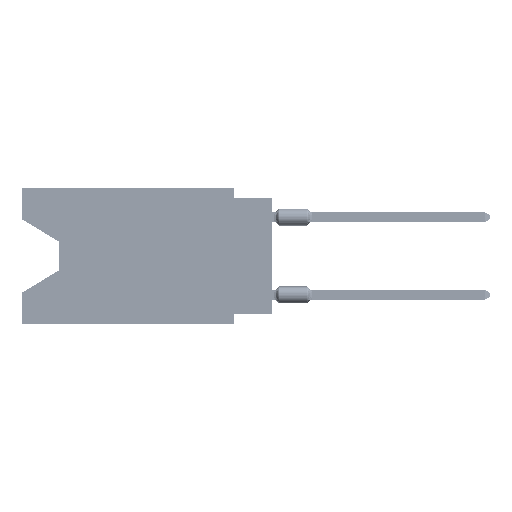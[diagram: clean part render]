
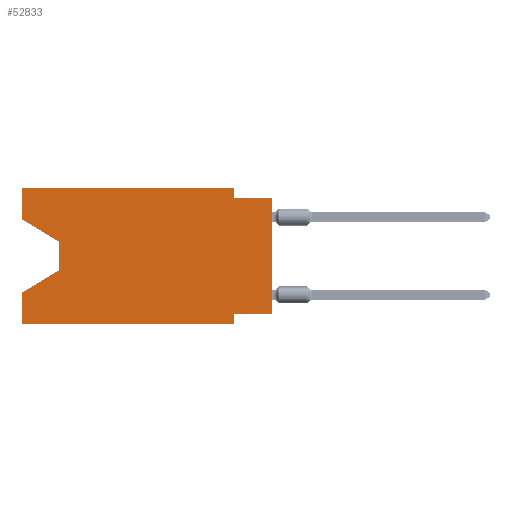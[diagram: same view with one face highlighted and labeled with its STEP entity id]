
A CAD part, left-side view. The second image highlights one B-rep face of the part: STEP entity #52833.
In plain terms, the highlighted planar face has unit normal (-1, 0, 0).
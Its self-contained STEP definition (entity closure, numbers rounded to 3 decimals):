
#71 = CARTESIAN_POINT ( 'NONE',  ( 0., 2.54, 0. ) ) ;
#236 = ORIENTED_EDGE ( 'NONE', *, *, #47545, .F. ) ;
#617 = VERTEX_POINT ( 'NONE', #4711 ) ;
#1688 = VECTOR ( 'NONE', #77916, 1000. ) ;
#2017 = EDGE_CURVE ( 'NONE', #23931, #95659, #14668, .T. ) ;
#2189 = LINE ( 'NONE', #18278, #55509 ) ;
#2536 = EDGE_CURVE ( 'NONE', #5876, #23931, #67046, .T. ) ;
#2810 = VECTOR ( 'NONE', #63174, 1000. ) ;
#3222 = VECTOR ( 'NONE', #25770, 1000. ) ;
#4711 = CARTESIAN_POINT ( 'NONE',  ( 0., 13.97, -5.385 ) ) ;
#5492 = EDGE_LOOP ( 'NONE', ( #47874, #43625, #38110, #98018, #96078, #26086, #236, #100570, #89663, #18626, #103654, #66525 ) ) ;
#5876 = VERTEX_POINT ( 'NONE', #17635 ) ;
#9688 = CARTESIAN_POINT ( 'NONE',  ( 0., 2.54, -8.89 ) ) ;
#13386 = CARTESIAN_POINT ( 'NONE',  ( 0., 16.383, 0. ) ) ;
#14668 = LINE ( 'NONE', #91004, #31913 ) ;
#17483 = CARTESIAN_POINT ( 'NONE',  ( 0., 0., -8.255 ) ) ;
#17635 = CARTESIAN_POINT ( 'NONE',  ( 0., 2.54, 0. ) ) ;
#18177 = CARTESIAN_POINT ( 'NONE',  ( 0., 16.383, -8.89 ) ) ;
#18278 = CARTESIAN_POINT ( 'NONE',  ( 0., 13.97, -3.505 ) ) ;
#18626 = ORIENTED_EDGE ( 'NONE', *, *, #2536, .F. ) ;
#18951 = EDGE_CURVE ( 'NONE', #60144, #62199, #61837, .T. ) ;
#20106 = EDGE_CURVE ( 'NONE', #58597, #37844, #100655, .T. ) ;
#23905 = DIRECTION ( 'NONE',  ( 0., 0., -1. ) ) ;
#23931 = VERTEX_POINT ( 'NONE', #105452 ) ;
#25770 = DIRECTION ( 'NONE',  ( 0., 1., 0. ) ) ;
#26086 = ORIENTED_EDGE ( 'NONE', *, *, #30663, .F. ) ;
#26466 = CARTESIAN_POINT ( 'NONE',  ( 0., 16.383, -8.89 ) ) ;
#26805 = VECTOR ( 'NONE', #23905, 1000. ) ;
#27050 = LINE ( 'NONE', #68543, #40132 ) ;
#29397 = CARTESIAN_POINT ( 'NONE',  ( 0., 2.54, -8.255 ) ) ;
#30663 = EDGE_CURVE ( 'NONE', #95774, #62199, #98749, .T. ) ;
#31913 = VECTOR ( 'NONE', #47823, 1000. ) ;
#33353 = LINE ( 'NONE', #104001, #107307 ) ;
#34605 = FACE_OUTER_BOUND ( 'NONE', #5492, .T. ) ;
#37103 = VECTOR ( 'NONE', #109056, 1000. ) ;
#37844 = VERTEX_POINT ( 'NONE', #72080 ) ;
#37937 = EDGE_CURVE ( 'NONE', #71720, #5876, #74787, .T. ) ;
#38110 = ORIENTED_EDGE ( 'NONE', *, *, #46682, .T. ) ;
#40132 = VECTOR ( 'NONE', #42532, 1000. ) ;
#41425 = CARTESIAN_POINT ( 'NONE',  ( 0., 16.383, -2.038 ) ) ;
#42532 = DIRECTION ( 'NONE',  ( 0., 0., 1. ) ) ;
#43625 = ORIENTED_EDGE ( 'NONE', *, *, #81643, .T. ) ;
#44349 = DIRECTION ( 'NONE',  ( 0., 0., 1. ) ) ;
#45270 = EDGE_CURVE ( 'NONE', #58597, #71720, #101950, .T. ) ;
#45352 = EDGE_CURVE ( 'NONE', #60144, #102202, #62618, .T. ) ;
#46682 = EDGE_CURVE ( 'NONE', #617, #102202, #33353, .T. ) ;
#47545 = EDGE_CURVE ( 'NONE', #88094, #95774, #102110, .T. ) ;
#47823 = DIRECTION ( 'NONE',  ( 0., -1., 0. ) ) ;
#47874 = ORIENTED_EDGE ( 'NONE', *, *, #20106, .T. ) ;
#48626 = VECTOR ( 'NONE', #107039, 1000. ) ;
#52265 = DIRECTION ( 'NONE',  ( 0., 0., -1. ) ) ;
#52610 = CARTESIAN_POINT ( 'NONE',  ( 0., 0., -0.635 ) ) ;
#52833 = ADVANCED_FACE ( 'NONE', ( #34605 ), #68364, .F. ) ;
#55509 = VECTOR ( 'NONE', #60842, 1000. ) ;
#57018 = CARTESIAN_POINT ( 'NONE',  ( 0., 16.383, -2.038 ) ) ;
#58597 = VERTEX_POINT ( 'NONE', #57018 ) ;
#60144 = VERTEX_POINT ( 'NONE', #26466 ) ;
#60842 = DIRECTION ( 'NONE',  ( 0., 0., -1. ) ) ;
#61684 = CARTESIAN_POINT ( 'NONE',  ( 0., 16.383, 0. ) ) ;
#61837 = LINE ( 'NONE', #18177, #1688 ) ;
#61964 = VECTOR ( 'NONE', #93445, 1000. ) ;
#62199 = VERTEX_POINT ( 'NONE', #9688 ) ;
#62618 = LINE ( 'NONE', #13386, #2810 ) ;
#63174 = DIRECTION ( 'NONE',  ( 0., 0., 1. ) ) ;
#66525 = ORIENTED_EDGE ( 'NONE', *, *, #45270, .F. ) ;
#67046 = LINE ( 'NONE', #71, #26805 ) ;
#68364 = PLANE ( 'NONE',  #105151 ) ;
#68543 = CARTESIAN_POINT ( 'NONE',  ( 0., 0., 0. ) ) ;
#71720 = VERTEX_POINT ( 'NONE', #96349 ) ;
#72080 = CARTESIAN_POINT ( 'NONE',  ( 0., 13.97, -3.505 ) ) ;
#74787 = LINE ( 'NONE', #75878, #37103 ) ;
#74946 = CARTESIAN_POINT ( 'NONE',  ( 0., 2.54, -8.89 ) ) ;
#75878 = CARTESIAN_POINT ( 'NONE',  ( 0., 16.383, 0. ) ) ;
#77916 = DIRECTION ( 'NONE',  ( 0., -1., 0. ) ) ;
#78020 = DIRECTION ( 'NONE',  ( 0., 0.855, -0.519 ) ) ;
#80073 = CARTESIAN_POINT ( 'NONE',  ( 0., 0., -8.255 ) ) ;
#81643 = EDGE_CURVE ( 'NONE', #37844, #617, #2189, .T. ) ;
#86619 = DIRECTION ( 'NONE',  ( 1., 0., 0. ) ) ;
#88094 = VERTEX_POINT ( 'NONE', #80073 ) ;
#89498 = VECTOR ( 'NONE', #44349, 1000. ) ;
#89663 = ORIENTED_EDGE ( 'NONE', *, *, #2017, .F. ) ;
#91004 = CARTESIAN_POINT ( 'NONE',  ( 0., 0., -0.635 ) ) ;
#93397 = EDGE_CURVE ( 'NONE', #88094, #95659, #27050, .T. ) ;
#93445 = DIRECTION ( 'NONE',  ( 0., -0.855, -0.519 ) ) ;
#95300 = CARTESIAN_POINT ( 'NONE',  ( 0., 16.383, 0. ) ) ;
#95659 = VERTEX_POINT ( 'NONE', #52610 ) ;
#95774 = VERTEX_POINT ( 'NONE', #29397 ) ;
#96078 = ORIENTED_EDGE ( 'NONE', *, *, #18951, .T. ) ;
#96349 = CARTESIAN_POINT ( 'NONE',  ( 0., 16.383, 0. ) ) ;
#98018 = ORIENTED_EDGE ( 'NONE', *, *, #45352, .F. ) ;
#98749 = LINE ( 'NONE', #74946, #48626 ) ;
#100518 = CARTESIAN_POINT ( 'NONE',  ( 0., 16.383, -6.852 ) ) ;
#100570 = ORIENTED_EDGE ( 'NONE', *, *, #93397, .T. ) ;
#100655 = LINE ( 'NONE', #41425, #61964 ) ;
#101950 = LINE ( 'NONE', #95300, #89498 ) ;
#102110 = LINE ( 'NONE', #17483, #3222 ) ;
#102202 = VERTEX_POINT ( 'NONE', #100518 ) ;
#103654 = ORIENTED_EDGE ( 'NONE', *, *, #37937, .F. ) ;
#104001 = CARTESIAN_POINT ( 'NONE',  ( 0., 13.97, -5.385 ) ) ;
#105151 = AXIS2_PLACEMENT_3D ( 'NONE', #61684, #86619, #52265 ) ;
#105452 = CARTESIAN_POINT ( 'NONE',  ( 0., 2.54, -0.635 ) ) ;
#107039 = DIRECTION ( 'NONE',  ( 0., 0., -1. ) ) ;
#107307 = VECTOR ( 'NONE', #78020, 1000. ) ;
#109056 = DIRECTION ( 'NONE',  ( 0., -1., 0. ) ) ;
